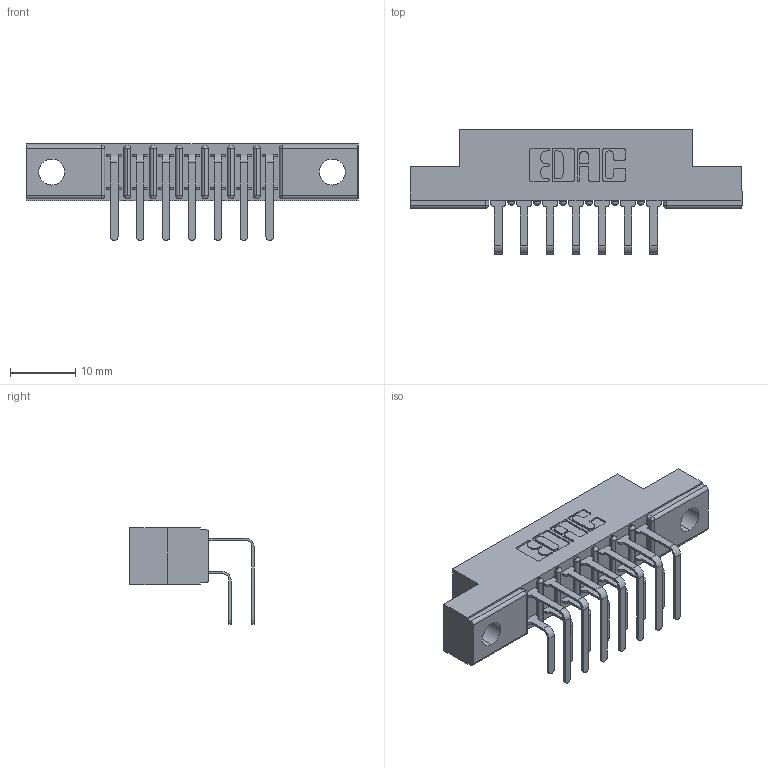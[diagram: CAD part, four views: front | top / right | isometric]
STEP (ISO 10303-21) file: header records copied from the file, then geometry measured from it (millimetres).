
FILE_DESCRIPTION (( 'STEP AP203' ), '1' );
FILE_NAME ('357-007-458-104.STEP', '2020-09-30T01:53:05', ( '' ), ( '' ), 'SwSTEP 2.0', 'SolidWorks 2020', '' );
FILE_SCHEMA (( 'CONFIG_CONTROL_DESIGN' ));
Length unit declared in the file: inch
Products named in the file (4): 307 Part_.156 Dia Mounting Holes; 357-007-458-104; 307-290-001_558 559 - 1 (Single); 307-290-001_558 - 2 (Single)
Assembly tree (15 placements, depth 2):
  357-007-458-104
    307 Part_.156 Dia Mounting Holes
    307-290-001_558 559 - 1 (Single)  x7
    307-290-001_558 - 2 (Single)  x7
Bounding box: 50.75 x 18.96 x 14.81 mm (x, y, z)
Volume: 3277.3 mm3; surface area: 5244.2 mm2
Topology: 15 solids, 15 shells, 840 faces, 2347 edges, 1522 vertices
Faces by surface type: plane 546, cylinder 278, sphere 16
Entity records: 12405 total; most frequent: CARTESIAN_POINT 2047, ORIENTED_EDGE 2022, DIRECTION 2011, EDGE_CURVE 1011, LINE 767, VECTOR 767, VERTEX_POINT 658, AXIS2_PLACEMENT_3D 622
